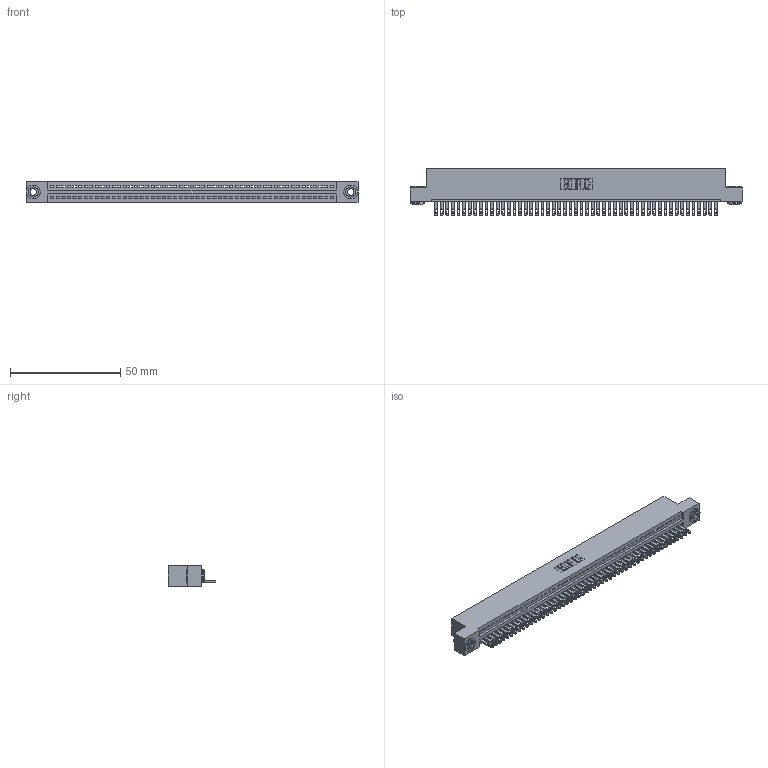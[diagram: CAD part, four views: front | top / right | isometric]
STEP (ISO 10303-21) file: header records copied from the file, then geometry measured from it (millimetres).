
FILE_DESCRIPTION (( 'STEP AP203' ), '1' );
FILE_NAME ('895-051-500-103.STEP', '2020-09-27T10:01:36', ( '' ), ( '' ), 'SwSTEP 2.0', 'SolidWorks 2020', '' );
FILE_SCHEMA (( 'CONFIG_CONTROL_DESIGN' ));
Length unit declared in the file: inch
Products named in the file (4): 845 Part_Flush Mounting Lugs - 0.156 Dia-TH; 345-250-002_345-250-002-102; 345-292-001_345-293-100; 895-051-500-103
Assembly tree (54 placements, depth 2):
  895-051-500-103
    845 Part_Flush Mounting Lugs - 0.156 Dia-TH
    345-292-001_345-293-100  x51
    345-250-002_345-250-002-102  x2
Bounding box: 150.75 x 21.51 x 9.4 mm (x, y, z)
Volume: 14443 mm3; surface area: 19644.7 mm2
Topology: 54 solids, 54 shells, 2918 faces, 8985 edges, 5986 vertices
Faces by surface type: plane 1824, cylinder 1086, cone 8
Entity records: 37752 total; most frequent: CARTESIAN_POINT 6516, ORIENTED_EDGE 6494, DIRECTION 5711, EDGE_CURVE 3247, LINE 2883, VECTOR 2883, VERTEX_POINT 2162, AXIS2_PLACEMENT_3D 1414
